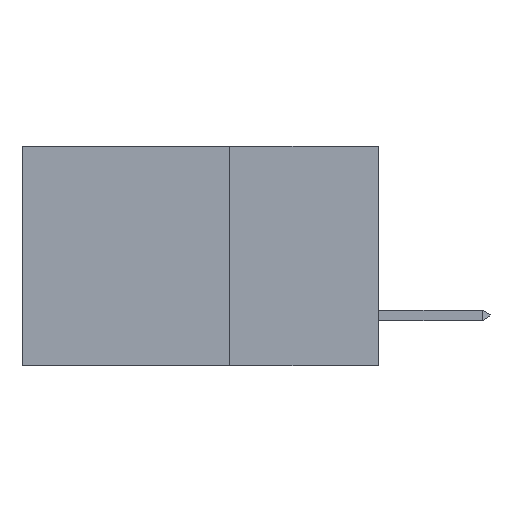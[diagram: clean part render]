
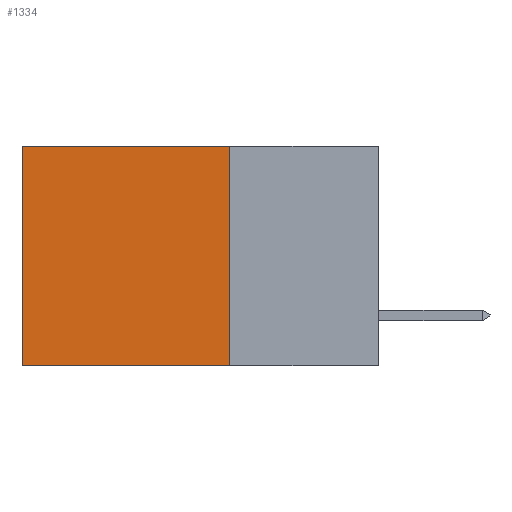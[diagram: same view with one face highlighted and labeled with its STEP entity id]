
A CAD part, left-side view. The second image highlights one B-rep face of the part: STEP entity #1334.
In plain terms, the highlighted planar face has unit normal (-1, 0, 0).
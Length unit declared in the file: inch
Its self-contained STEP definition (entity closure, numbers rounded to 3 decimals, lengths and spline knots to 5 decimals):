
#205 = ORIENTED_EDGE ( 'NONE', *, *, #11991, .F. ) ;
#682 = VECTOR ( 'NONE', #11715, 39.37008 ) ;
#747 = PLANE ( 'NONE',  #6861 ) ;
#822 = VERTEX_POINT ( 'NONE', #5464 ) ;
#1334 = ADVANCED_FACE ( 'NONE', ( #13832 ), #747, .F. ) ;
#1573 = EDGE_CURVE ( 'NONE', #6717, #5484, #14589, .T. ) ;
#2676 = VECTOR ( 'NONE', #12503, 39.37008 ) ;
#3685 = VECTOR ( 'NONE', #5956, 39.37008 ) ;
#3989 = VECTOR ( 'NONE', #8537, 39.37008 ) ;
#5404 = EDGE_CURVE ( 'NONE', #11880, #6717, #8453, .T. ) ;
#5464 = CARTESIAN_POINT ( 'NONE',  ( 0.298, 0.25, -0.37 ) ) ;
#5484 = VERTEX_POINT ( 'NONE', #14022 ) ;
#5759 = CARTESIAN_POINT ( 'NONE',  ( 0.298, 0.25, 0. ) ) ;
#5956 = DIRECTION ( 'NONE',  ( 0., 0., -1. ) ) ;
#6416 = ORIENTED_EDGE ( 'NONE', *, *, #5404, .T. ) ;
#6717 = VERTEX_POINT ( 'NONE', #10649 ) ;
#6861 = AXIS2_PLACEMENT_3D ( 'NONE', #5759, #14391, #10436 ) ;
#8278 = LINE ( 'NONE', #14537, #3685 ) ;
#8453 = LINE ( 'NONE', #13550, #2676 ) ;
#8510 = ORIENTED_EDGE ( 'NONE', *, *, #9599, .F. ) ;
#8537 = DIRECTION ( 'NONE',  ( 0., 1., 0. ) ) ;
#9599 = EDGE_CURVE ( 'NONE', #11880, #822, #8278, .T. ) ;
#10436 = DIRECTION ( 'NONE',  ( 0., 0., -1. ) ) ;
#10520 = CARTESIAN_POINT ( 'NONE',  ( 0.298, 0.6, 0. ) ) ;
#10649 = CARTESIAN_POINT ( 'NONE',  ( 0.298, 0.6, 0. ) ) ;
#10894 = LINE ( 'NONE', #14811, #3989 ) ;
#11681 = EDGE_LOOP ( 'NONE', ( #15362, #205, #8510, #6416 ) ) ;
#11715 = DIRECTION ( 'NONE',  ( 0., 0., -1. ) ) ;
#11880 = VERTEX_POINT ( 'NONE', #11956 ) ;
#11956 = CARTESIAN_POINT ( 'NONE',  ( 0.298, 0.25, 0. ) ) ;
#11991 = EDGE_CURVE ( 'NONE', #822, #5484, #10894, .T. ) ;
#12503 = DIRECTION ( 'NONE',  ( 0., 1., 0. ) ) ;
#13550 = CARTESIAN_POINT ( 'NONE',  ( 0.298, 0.25, 0. ) ) ;
#13832 = FACE_OUTER_BOUND ( 'NONE', #11681, .T. ) ;
#14022 = CARTESIAN_POINT ( 'NONE',  ( 0.298, 0.6, -0.37 ) ) ;
#14391 = DIRECTION ( 'NONE',  ( 1., 0., 0. ) ) ;
#14537 = CARTESIAN_POINT ( 'NONE',  ( 0.298, 0.25, 0. ) ) ;
#14589 = LINE ( 'NONE', #10520, #682 ) ;
#14811 = CARTESIAN_POINT ( 'NONE',  ( 0.298, 0.25, -0.37 ) ) ;
#15362 = ORIENTED_EDGE ( 'NONE', *, *, #1573, .T. ) ;
